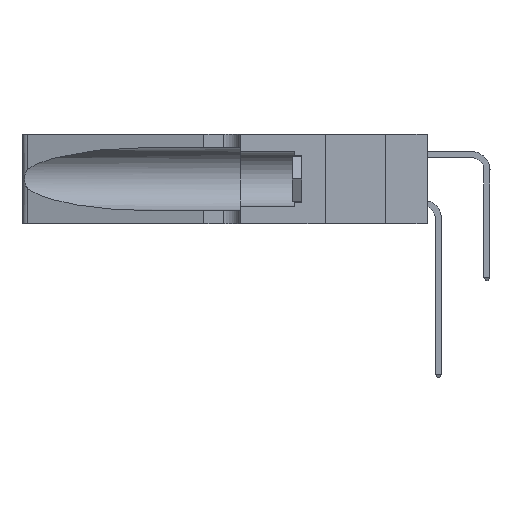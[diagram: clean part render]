
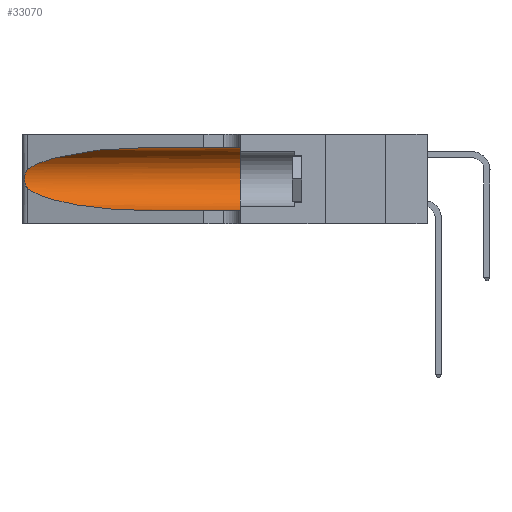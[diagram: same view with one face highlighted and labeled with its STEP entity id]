
A CAD part, left-side view. The second image highlights one B-rep face of the part: STEP entity #33070.
In plain terms, the highlighted cylindrical face has radius 3.308 mm (diameter 6.617 mm), a partial arc.
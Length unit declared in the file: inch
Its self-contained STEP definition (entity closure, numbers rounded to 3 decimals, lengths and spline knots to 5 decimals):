
#1566 = CARTESIAN_POINT ( 'NONE',  ( 0.25487, 1.22718, 0.14631 ) ) ;
#4140 = CARTESIAN_POINT ( 'NONE',  ( 0.2373, 1.15595, 0.28018 ) ) ;
#4916 = CARTESIAN_POINT ( 'NONE',  ( 0.25787, 1.23484, 0.2124 ) ) ;
#5171 = DIRECTION ( 'NONE',  ( 0., 0., 1. ) ) ;
#5231 = CARTESIAN_POINT ( 'NONE',  ( 0.18966, 0.96281, 0.05475 ) ) ;
#7427 = CARTESIAN_POINT ( 'NONE',  ( 0.1305, 0.72297, 0.05475 ) ) ;
#8687 = B_SPLINE_CURVE_WITH_KNOTS ( 'NONE', 3,
 ( #39530, #33587, #14317, #4916, #24308, #27545, #27413, #17366, #21069, #36680, #23874, #36963, #14577, #30874 ),
 .UNSPECIFIED., .F., .F.,
 ( 4, 2, 2, 2, 2, 2, 4 ),
 ( 0., 0.00027, 0.00053, 0.00107, 0.0016, 0.00187, 0.00214 ),
 .UNSPECIFIED. ) ;
#9285 = VERTEX_POINT ( 'NONE', #19333 ) ;
#10567 = CARTESIAN_POINT ( 'NONE',  ( 0.25487, 1.22718, 0.22369 ) ) ;
#10753 =( BOUNDED_CURVE ( )  B_SPLINE_CURVE ( 3, ( #14983, #39713, #4140, #36046 ),
 .UNSPECIFIED., .F., .F. ) 
 B_SPLINE_CURVE_WITH_KNOTS ( ( 4, 4 ),
 ( 1.5708, 2.84003 ),
 .UNSPECIFIED. ) 
 CURVE ( )  GEOMETRIC_REPRESENTATION_ITEM ( )  RATIONAL_B_SPLINE_CURVE ( ( 1., 0.87, 0.87, 1. ) ) 
 REPRESENTATION_ITEM ( '' )  );
#11003 = VECTOR ( 'NONE', #23928, 39.37008 ) ;
#12525 = CARTESIAN_POINT ( 'NONE',  ( 0.1305, 0.72297, 0.31525 ) ) ;
#13232 = VERTEX_POINT ( 'NONE', #25876 ) ;
#13488 = ORIENTED_EDGE ( 'NONE', *, *, #19519, .T. ) ;
#14190 = ORIENTED_EDGE ( 'NONE', *, *, #24353, .T. ) ;
#14317 = CARTESIAN_POINT ( 'NONE',  ( 0.25639, 1.23184, 0.21858 ) ) ;
#14577 = CARTESIAN_POINT ( 'NONE',  ( 0.25555, 1.22993, 0.14849 ) ) ;
#14983 = CARTESIAN_POINT ( 'NONE',  ( 0.1305, 0.72297, 0.31525 ) ) ;
#16560 = AXIS2_PLACEMENT_3D ( 'NONE', #17755, #17620, #5171 ) ;
#17366 = CARTESIAN_POINT ( 'NONE',  ( 0.26075, 1.23896, 0.178 ) ) ;
#17620 = DIRECTION ( 'NONE',  ( 0., 1., 0. ) ) ;
#17735 = EDGE_CURVE ( 'NONE', #36263, #26499, #10753, .T. ) ;
#17755 = CARTESIAN_POINT ( 'NONE',  ( 0.1305, 0.35, 0.185 ) ) ;
#18615 = VERTEX_POINT ( 'NONE', #21616 ) ;
#19333 = CARTESIAN_POINT ( 'NONE',  ( 0.1305, 0.35, 0.31525 ) ) ;
#19519 = EDGE_CURVE ( 'NONE', #23006, #13232, #37548, .T. ) ;
#19535 = ORIENTED_EDGE ( 'NONE', *, *, #30847, .F. ) ;
#20006 = EDGE_CURVE ( 'NONE', #36263, #9285, #31025, .T. ) ;
#20885 = DIRECTION ( 'NONE',  ( 0., -1., 0. ) ) ;
#20956 = CARTESIAN_POINT ( 'NONE',  ( 0.1305, 0.72297, 0.05475 ) ) ;
#21069 = CARTESIAN_POINT ( 'NONE',  ( 0.26017, 1.23833, 0.17102 ) ) ;
#21096 = CARTESIAN_POINT ( 'NONE',  ( 0.2373, 1.15595, 0.08982 ) ) ;
#21616 = CARTESIAN_POINT ( 'NONE',  ( 0.25487, 1.22718, 0.14631 ) ) ;
#23006 = VERTEX_POINT ( 'NONE', #7427 ) ;
#23695 = CARTESIAN_POINT ( 'NONE',  ( 0.1305, 1.61858, 0.31525 ) ) ;
#23874 = CARTESIAN_POINT ( 'NONE',  ( 0.25789, 1.23486, 0.15765 ) ) ;
#23928 = DIRECTION ( 'NONE',  ( 0., -1., 0. ) ) ;
#24308 = CARTESIAN_POINT ( 'NONE',  ( 0.25854, 1.2359, 0.20912 ) ) ;
#24353 = EDGE_CURVE ( 'NONE', #18615, #23006, #37665, .T. ) ;
#24894 = CIRCLE ( 'NONE', #16560, 0.13025 ) ;
#25465 = DIRECTION ( 'NONE',  ( 0., -1., 0. ) ) ;
#25485 = ORIENTED_EDGE ( 'NONE', *, *, #20006, .F. ) ;
#25876 = CARTESIAN_POINT ( 'NONE',  ( 0.1305, 0.35, 0.05475 ) ) ;
#26499 = VERTEX_POINT ( 'NONE', #10567 ) ;
#27413 = CARTESIAN_POINT ( 'NONE',  ( 0.26075, 1.23896, 0.19203 ) ) ;
#27545 = CARTESIAN_POINT ( 'NONE',  ( 0.26018, 1.23835, 0.19895 ) ) ;
#28720 = DIRECTION ( 'NONE',  ( 0., 0., -1. ) ) ;
#28758 = ORIENTED_EDGE ( 'NONE', *, *, #17735, .T. ) ;
#29479 = EDGE_CURVE ( 'NONE', #26499, #18615, #8687, .T. ) ;
#30847 = EDGE_CURVE ( 'NONE', #9285, #13232, #24894, .T. ) ;
#30874 = CARTESIAN_POINT ( 'NONE',  ( 0.25487, 1.22718, 0.14631 ) ) ;
#31025 = LINE ( 'NONE', #23695, #33475 ) ;
#31923 = ORIENTED_EDGE ( 'NONE', *, *, #29479, .T. ) ;
#33070 = ADVANCED_FACE ( 'NONE', ( #40634 ), #38566, .F. ) ;
#33475 = VECTOR ( 'NONE', #20885, 39.37008 ) ;
#33587 = CARTESIAN_POINT ( 'NONE',  ( 0.25555, 1.22994, 0.2215 ) ) ;
#35634 = EDGE_LOOP ( 'NONE', ( #28758, #31923, #14190, #13488, #19535, #25485 ) ) ;
#36046 = CARTESIAN_POINT ( 'NONE',  ( 0.25487, 1.22718, 0.22369 ) ) ;
#36263 = VERTEX_POINT ( 'NONE', #12525 ) ;
#36449 = AXIS2_PLACEMENT_3D ( 'NONE', #38641, #25465, #28720 ) ;
#36680 = CARTESIAN_POINT ( 'NONE',  ( 0.25856, 1.23593, 0.16098 ) ) ;
#36963 = CARTESIAN_POINT ( 'NONE',  ( 0.25639, 1.23186, 0.15144 ) ) ;
#37548 = LINE ( 'NONE', #39977, #11003 ) ;
#37665 =( BOUNDED_CURVE ( )  B_SPLINE_CURVE ( 3, ( #1566, #21096, #5231, #20956 ),
 .UNSPECIFIED., .F., .F. ) 
 B_SPLINE_CURVE_WITH_KNOTS ( ( 4, 4 ),
 ( 3.44316, 4.71239 ),
 .UNSPECIFIED. ) 
 CURVE ( )  GEOMETRIC_REPRESENTATION_ITEM ( )  RATIONAL_B_SPLINE_CURVE ( ( 1., 0.87, 0.87, 1. ) ) 
 REPRESENTATION_ITEM ( '' )  );
#38566 = CYLINDRICAL_SURFACE ( 'NONE', #36449, 0.13025 ) ;
#38641 = CARTESIAN_POINT ( 'NONE',  ( 0.1305, 1.61858, 0.185 ) ) ;
#39530 = CARTESIAN_POINT ( 'NONE',  ( 0.25487, 1.22718, 0.22369 ) ) ;
#39713 = CARTESIAN_POINT ( 'NONE',  ( 0.18966, 0.96281, 0.31525 ) ) ;
#39977 = CARTESIAN_POINT ( 'NONE',  ( 0.1305, 1.61858, 0.05475 ) ) ;
#40634 = FACE_OUTER_BOUND ( 'NONE', #35634, .T. ) ;
